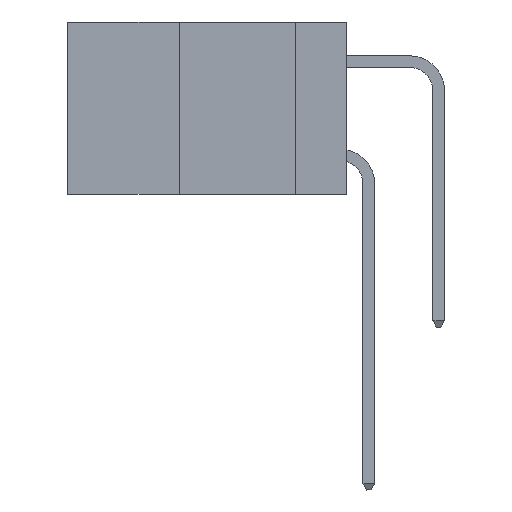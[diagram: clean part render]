
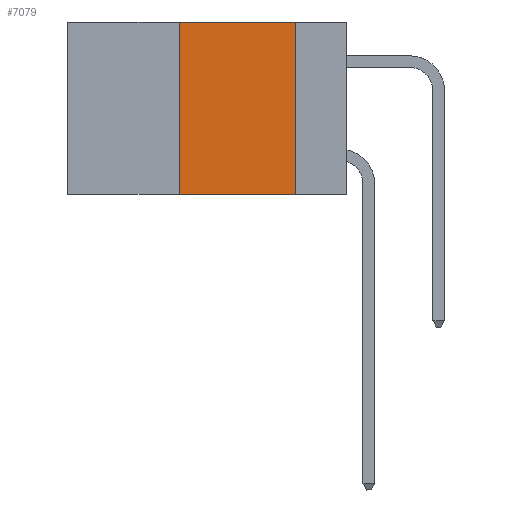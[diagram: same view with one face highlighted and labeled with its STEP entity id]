
A CAD part, left-side view. The second image highlights one B-rep face of the part: STEP entity #7079.
In plain terms, the highlighted planar face has unit normal (-1, 0, 0).
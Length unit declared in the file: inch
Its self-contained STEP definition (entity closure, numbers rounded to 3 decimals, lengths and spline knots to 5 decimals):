
#117 = VECTOR ( 'NONE', #6920, 39.37008 ) ;
#258 = CARTESIAN_POINT ( 'NONE',  ( 0., 0.36, 0. ) ) ;
#533 = CARTESIAN_POINT ( 'NONE',  ( 0., 0.6, -0.37 ) ) ;
#1047 = ORIENTED_EDGE ( 'NONE', *, *, #3059, .F. ) ;
#1129 = EDGE_CURVE ( 'NONE', #1840, #1408, #7472, .T. ) ;
#1408 = VERTEX_POINT ( 'NONE', #5308 ) ;
#1840 = VERTEX_POINT ( 'NONE', #10781 ) ;
#1919 = EDGE_CURVE ( 'NONE', #4732, #1408, #8042, .T. ) ;
#2445 = CARTESIAN_POINT ( 'NONE',  ( 0., 0.6, 0. ) ) ;
#2665 = VECTOR ( 'NONE', #4542, 39.37008 ) ;
#3014 = EDGE_LOOP ( 'NONE', ( #6289, #5650, #1047, #10441 ) ) ;
#3059 = EDGE_CURVE ( 'NONE', #4732, #8081, #10673, .T. ) ;
#3280 = DIRECTION ( 'NONE',  ( 1., 0., 0. ) ) ;
#3633 = VECTOR ( 'NONE', #7815, 39.37008 ) ;
#4542 = DIRECTION ( 'NONE',  ( 0., 0., -1. ) ) ;
#4732 = VERTEX_POINT ( 'NONE', #6459 ) ;
#5308 = CARTESIAN_POINT ( 'NONE',  ( 0., 0.11, -0.37 ) ) ;
#5650 = ORIENTED_EDGE ( 'NONE', *, *, #9040, .F. ) ;
#6069 = PLANE ( 'NONE',  #9800 ) ;
#6289 = ORIENTED_EDGE ( 'NONE', *, *, #1129, .F. ) ;
#6459 = CARTESIAN_POINT ( 'NONE',  ( 0., 0.36, -0.37 ) ) ;
#6630 = VECTOR ( 'NONE', #11563, 39.37008 ) ;
#6920 = DIRECTION ( 'NONE',  ( 0., 0., 1. ) ) ;
#7079 = ADVANCED_FACE ( 'NONE', ( #7806 ), #6069, .F. ) ;
#7472 = LINE ( 'NONE', #11156, #2665 ) ;
#7806 = FACE_OUTER_BOUND ( 'NONE', #3014, .T. ) ;
#7815 = DIRECTION ( 'NONE',  ( 0., -1., 0. ) ) ;
#8042 = LINE ( 'NONE', #533, #3633 ) ;
#8081 = VERTEX_POINT ( 'NONE', #258 ) ;
#9040 = EDGE_CURVE ( 'NONE', #8081, #1840, #10595, .T. ) ;
#9800 = AXIS2_PLACEMENT_3D ( 'NONE', #11569, #3280, #11504 ) ;
#10441 = ORIENTED_EDGE ( 'NONE', *, *, #1919, .T. ) ;
#10595 = LINE ( 'NONE', #2445, #6630 ) ;
#10673 = LINE ( 'NONE', #11693, #117 ) ;
#10781 = CARTESIAN_POINT ( 'NONE',  ( 0., 0.11, 0. ) ) ;
#11156 = CARTESIAN_POINT ( 'NONE',  ( 0., 0.11, 0. ) ) ;
#11504 = DIRECTION ( 'NONE',  ( 0., 0., -1. ) ) ;
#11563 = DIRECTION ( 'NONE',  ( 0., -1., 0. ) ) ;
#11569 = CARTESIAN_POINT ( 'NONE',  ( 0., 0.6, 0. ) ) ;
#11693 = CARTESIAN_POINT ( 'NONE',  ( 0., 0.36, 0. ) ) ;
